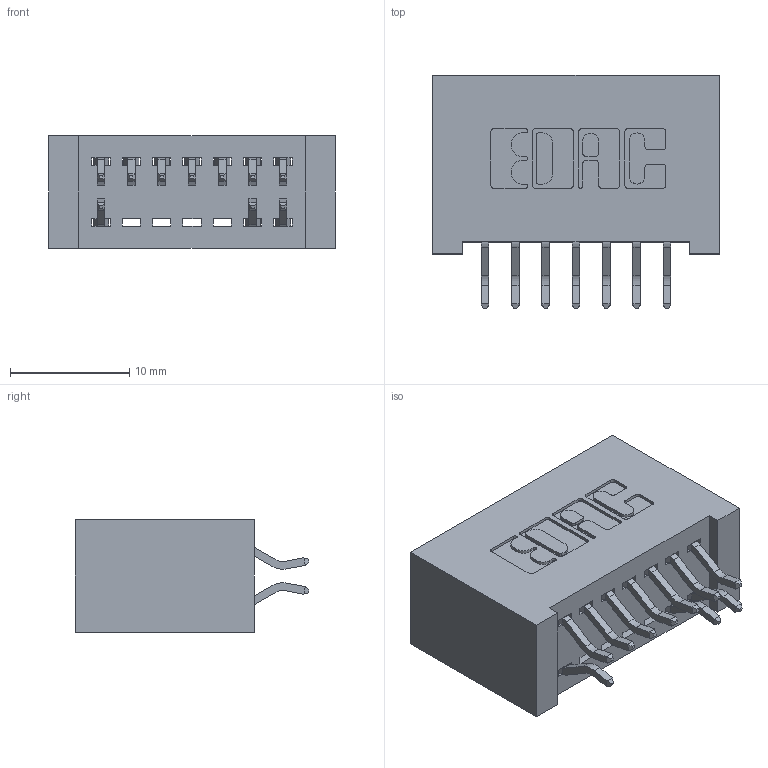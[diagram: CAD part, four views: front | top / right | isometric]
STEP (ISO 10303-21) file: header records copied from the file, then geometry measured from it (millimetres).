
FILE_DESCRIPTION (( 'STEP AP203' ), '1' );
FILE_NAME ('392-014-556-201.STEP', '2018-08-15T00:20:02', ( '' ), ( '' ), 'SwSTEP 2.0', 'SolidWorks 2016', '' );
FILE_SCHEMA (( 'CONFIG_CONTROL_DESIGN' ));
Length unit declared in the file: inch
Products named in the file (3): 392-014-556-201; 342 Part_Lugless; 345-292-001_556 Tail
Assembly tree (11 placements, depth 2):
  392-014-556-201
    342 Part_Lugless
    345-292-001_556 Tail  x10
Bounding box: 24.03 x 19.58 x 9.4 mm (x, y, z)
Volume: 2396.5 mm3; surface area: 3276.1 mm2
Topology: 11 solids, 11 shells, 706 faces, 2089 edges, 1378 vertices
Faces by surface type: plane 486, cylinder 220
Entity records: 8713 total; most frequent: CARTESIAN_POINT 1514, ORIENTED_EDGE 1442, DIRECTION 1333, EDGE_CURVE 721, LINE 593, VECTOR 593, VERTEX_POINT 478, AXIS2_PLACEMENT_3D 370
